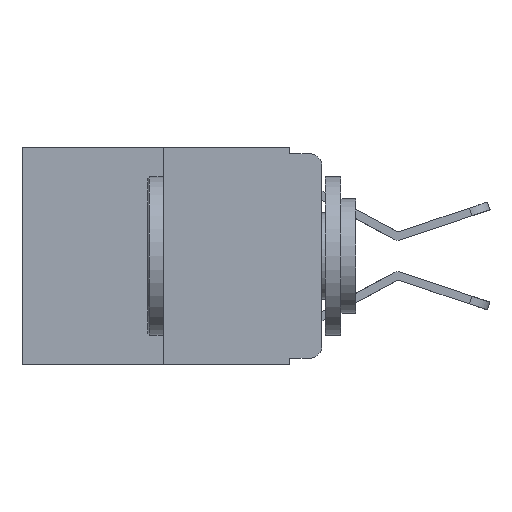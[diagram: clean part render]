
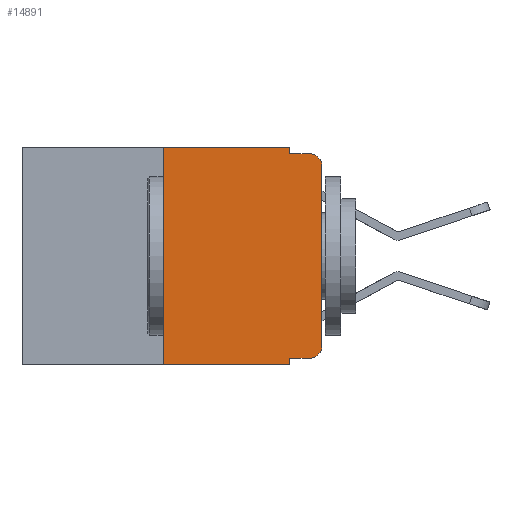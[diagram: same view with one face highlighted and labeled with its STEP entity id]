
A CAD part, left-side view. The second image highlights one B-rep face of the part: STEP entity #14891.
In plain terms, the highlighted planar face has unit normal (-1, 0, 0).
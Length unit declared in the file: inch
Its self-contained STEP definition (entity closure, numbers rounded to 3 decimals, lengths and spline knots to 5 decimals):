
#174 = DIRECTION ( 'NONE',  ( 0., 0., -1. ) ) ;
#260 = AXIS2_PLACEMENT_3D ( 'NONE', #15573, #7341, #16896 ) ;
#284 = ORIENTED_EDGE ( 'NONE', *, *, #13036, .F. ) ;
#495 = EDGE_LOOP ( 'NONE', ( #5687, #3307, #14386, #7873, #12084, #284, #14032, #1844, #17559, #4273 ) ) ;
#770 = DIRECTION ( 'NONE',  ( 0., 0., -1. ) ) ;
#787 = CARTESIAN_POINT ( 'NONE',  ( 0., 0., -0.03 ) ) ;
#1844 = ORIENTED_EDGE ( 'NONE', *, *, #17411, .F. ) ;
#2080 = CARTESIAN_POINT ( 'NONE',  ( 0., 0.473, -0.343 ) ) ;
#2511 = VERTEX_POINT ( 'NONE', #787 ) ;
#2562 = EDGE_CURVE ( 'NONE', #7000, #6347, #4528, .T. ) ;
#2906 = DIRECTION ( 'NONE',  ( 0., 0., -1. ) ) ;
#2978 = CARTESIAN_POINT ( 'NONE',  ( 0., 0.051, -0.01 ) ) ;
#3307 = ORIENTED_EDGE ( 'NONE', *, *, #15293, .T. ) ;
#3375 = CIRCLE ( 'NONE', #260, 0.02 ) ;
#3953 = VERTEX_POINT ( 'NONE', #5744 ) ;
#4201 = DIRECTION ( 'NONE',  ( 0., -1., 0. ) ) ;
#4249 = VECTOR ( 'NONE', #13741, 39.37008 ) ;
#4273 = ORIENTED_EDGE ( 'NONE', *, *, #6109, .T. ) ;
#4345 = LINE ( 'NONE', #16460, #7168 ) ;
#4528 = LINE ( 'NONE', #7747, #15125 ) ;
#4745 = VERTEX_POINT ( 'NONE', #10607 ) ;
#4768 = EDGE_CURVE ( 'NONE', #6347, #3953, #16695, .T. ) ;
#5092 = DIRECTION ( 'NONE',  ( 0., 0., 1. ) ) ;
#5313 = VECTOR ( 'NONE', #4201, 39.37008 ) ;
#5406 = CARTESIAN_POINT ( 'NONE',  ( 0., 0.25, 0. ) ) ;
#5484 = CARTESIAN_POINT ( 'NONE',  ( 0., 0.25, -0.343 ) ) ;
#5542 = AXIS2_PLACEMENT_3D ( 'NONE', #16225, #8032, #17552 ) ;
#5667 = VERTEX_POINT ( 'NONE', #8486 ) ;
#5687 = ORIENTED_EDGE ( 'NONE', *, *, #12922, .T. ) ;
#5744 = CARTESIAN_POINT ( 'NONE',  ( 0., 0.02, -0.01 ) ) ;
#6109 = EDGE_CURVE ( 'NONE', #11278, #5667, #13278, .T. ) ;
#6132 = EDGE_CURVE ( 'NONE', #4745, #11278, #16411, .T. ) ;
#6298 = CARTESIAN_POINT ( 'NONE',  ( 0., 0.02, -0.333 ) ) ;
#6347 = VERTEX_POINT ( 'NONE', #8517 ) ;
#6417 = LINE ( 'NONE', #6571, #12936 ) ;
#6571 = CARTESIAN_POINT ( 'NONE',  ( 0., 0., 0. ) ) ;
#6590 = AXIS2_PLACEMENT_3D ( 'NONE', #17259, #9131, #770 ) ;
#7000 = VERTEX_POINT ( 'NONE', #14287 ) ;
#7056 = VERTEX_POINT ( 'NONE', #15786 ) ;
#7168 = VECTOR ( 'NONE', #8296, 39.37008 ) ;
#7341 = DIRECTION ( 'NONE',  ( -1., 0., 0. ) ) ;
#7747 = CARTESIAN_POINT ( 'NONE',  ( 0., 0.051, 0. ) ) ;
#7873 = ORIENTED_EDGE ( 'NONE', *, *, #2562, .F. ) ;
#7932 = LINE ( 'NONE', #2080, #15247 ) ;
#7942 = LINE ( 'NONE', #5406, #4249 ) ;
#8032 = DIRECTION ( 'NONE',  ( -1., 0., 0. ) ) ;
#8296 = DIRECTION ( 'NONE',  ( 0., -1., 0. ) ) ;
#8486 = CARTESIAN_POINT ( 'NONE',  ( 0., 0., -0.313 ) ) ;
#8517 = CARTESIAN_POINT ( 'NONE',  ( 0., 0.051, -0.01 ) ) ;
#9131 = DIRECTION ( 'NONE',  ( 1., 0., 0. ) ) ;
#9164 = VECTOR ( 'NONE', #9431, 39.37008 ) ;
#9431 = DIRECTION ( 'NONE',  ( 0., -1., 0. ) ) ;
#9533 = VERTEX_POINT ( 'NONE', #5484 ) ;
#9960 = CARTESIAN_POINT ( 'NONE',  ( 0., 0.051, 0. ) ) ;
#10254 = EDGE_CURVE ( 'NONE', #15692, #7000, #4345, .T. ) ;
#10389 = CARTESIAN_POINT ( 'NONE',  ( 0., 0.25, 0. ) ) ;
#10607 = CARTESIAN_POINT ( 'NONE',  ( 0., 0.051, -0.333 ) ) ;
#10835 = CARTESIAN_POINT ( 'NONE',  ( 0., 0.051, -0.333 ) ) ;
#11155 = VECTOR ( 'NONE', #174, 39.37008 ) ;
#11278 = VERTEX_POINT ( 'NONE', #6298 ) ;
#11851 = DIRECTION ( 'NONE',  ( 0., -1., 0. ) ) ;
#12084 = ORIENTED_EDGE ( 'NONE', *, *, #10254, .F. ) ;
#12650 = FACE_OUTER_BOUND ( 'NONE', #495, .T. ) ;
#12922 = EDGE_CURVE ( 'NONE', #5667, #2511, #6417, .T. ) ;
#12936 = VECTOR ( 'NONE', #5092, 39.37008 ) ;
#13036 = EDGE_CURVE ( 'NONE', #9533, #15692, #7942, .T. ) ;
#13278 = CIRCLE ( 'NONE', #5542, 0.02 ) ;
#13741 = DIRECTION ( 'NONE',  ( 0., 0., 1. ) ) ;
#14032 = ORIENTED_EDGE ( 'NONE', *, *, #15690, .T. ) ;
#14287 = CARTESIAN_POINT ( 'NONE',  ( 0., 0.051, 0. ) ) ;
#14386 = ORIENTED_EDGE ( 'NONE', *, *, #4768, .F. ) ;
#14620 = PLANE ( 'NONE',  #6590 ) ;
#14891 = ADVANCED_FACE ( 'NONE', ( #12650 ), #14620, .F. ) ;
#15125 = VECTOR ( 'NONE', #2906, 39.37008 ) ;
#15247 = VECTOR ( 'NONE', #11851, 39.37008 ) ;
#15293 = EDGE_CURVE ( 'NONE', #2511, #3953, #3375, .T. ) ;
#15573 = CARTESIAN_POINT ( 'NONE',  ( 0., 0.02, -0.03 ) ) ;
#15690 = EDGE_CURVE ( 'NONE', #9533, #7056, #7932, .T. ) ;
#15692 = VERTEX_POINT ( 'NONE', #10389 ) ;
#15786 = CARTESIAN_POINT ( 'NONE',  ( 0., 0.051, -0.343 ) ) ;
#16225 = CARTESIAN_POINT ( 'NONE',  ( 0., 0.02, -0.313 ) ) ;
#16411 = LINE ( 'NONE', #10835, #9164 ) ;
#16460 = CARTESIAN_POINT ( 'NONE',  ( 0., 0.473, 0. ) ) ;
#16695 = LINE ( 'NONE', #2978, #5313 ) ;
#16896 = DIRECTION ( 'NONE',  ( 0., 0., -1. ) ) ;
#17259 = CARTESIAN_POINT ( 'NONE',  ( 0., 0.473, 0. ) ) ;
#17411 = EDGE_CURVE ( 'NONE', #4745, #7056, #17866, .T. ) ;
#17552 = DIRECTION ( 'NONE',  ( 0., 0., -1. ) ) ;
#17559 = ORIENTED_EDGE ( 'NONE', *, *, #6132, .T. ) ;
#17866 = LINE ( 'NONE', #9960, #11155 ) ;
